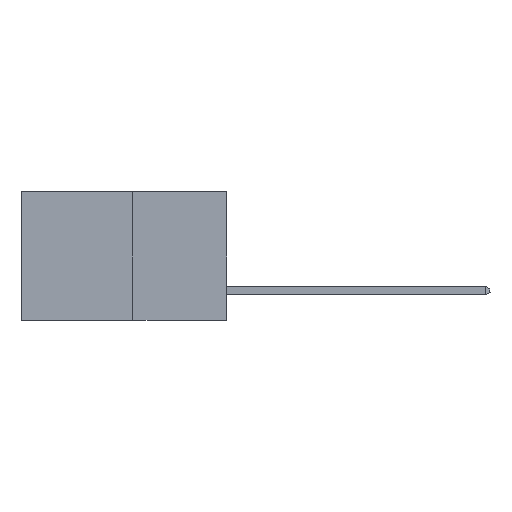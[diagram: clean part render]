
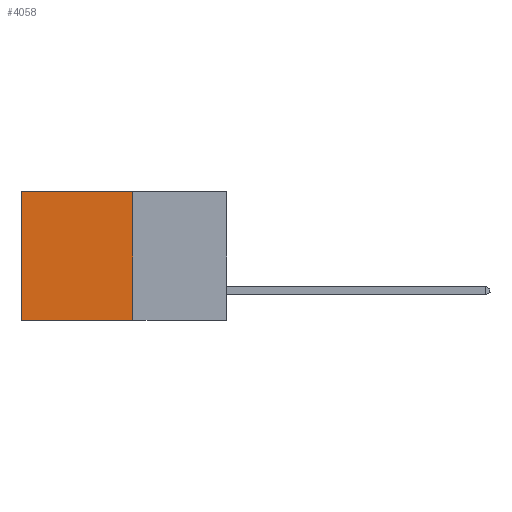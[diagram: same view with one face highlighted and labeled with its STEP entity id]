
A CAD part, left-side view. The second image highlights one B-rep face of the part: STEP entity #4058.
In plain terms, the highlighted planar face has unit normal (-1, 0, 0).
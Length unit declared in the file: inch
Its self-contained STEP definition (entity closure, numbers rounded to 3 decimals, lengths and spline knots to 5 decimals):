
#141 = CARTESIAN_POINT ( 'NONE',  ( 0.277, 0.59, 0. ) ) ;
#2171 = CARTESIAN_POINT ( 'NONE',  ( 0.277, 0.27, 0. ) ) ;
#2784 = VECTOR ( 'NONE', #7173, 39.37008 ) ;
#4058 = ADVANCED_FACE ( 'NONE', ( #8929 ), #28947, .F. ) ;
#4300 = EDGE_CURVE ( 'NONE', #28720, #6236, #8513, .T. ) ;
#4923 = ORIENTED_EDGE ( 'NONE', *, *, #13989, .T. ) ;
#6236 = VERTEX_POINT ( 'NONE', #17850 ) ;
#7173 = DIRECTION ( 'NONE',  ( 0., 1., 0. ) ) ;
#7540 = DIRECTION ( 'NONE',  ( 0., 0., -1. ) ) ;
#7547 = DIRECTION ( 'NONE',  ( 1., 0., 0. ) ) ;
#8355 = VECTOR ( 'NONE', #17525, 39.37008 ) ;
#8513 = LINE ( 'NONE', #13047, #2784 ) ;
#8929 = FACE_OUTER_BOUND ( 'NONE', #14458, .T. ) ;
#8979 = VECTOR ( 'NONE', #29089, 39.37008 ) ;
#9143 = LINE ( 'NONE', #15182, #8355 ) ;
#9300 = ORIENTED_EDGE ( 'NONE', *, *, #25645, .F. ) ;
#11284 = VECTOR ( 'NONE', #19034, 39.37008 ) ;
#11426 = ORIENTED_EDGE ( 'NONE', *, *, #22081, .T. ) ;
#13047 = CARTESIAN_POINT ( 'NONE',  ( 0.277, 0.27, -0.37 ) ) ;
#13196 = VERTEX_POINT ( 'NONE', #141 ) ;
#13989 = EDGE_CURVE ( 'NONE', #19200, #13196, #30146, .T. ) ;
#14458 = EDGE_LOOP ( 'NONE', ( #11426, #21713, #9300, #4923 ) ) ;
#15182 = CARTESIAN_POINT ( 'NONE',  ( 0.277, 0.59, -0.37 ) ) ;
#15570 = CARTESIAN_POINT ( 'NONE',  ( 0.277, 0.27, -0.37 ) ) ;
#17525 = DIRECTION ( 'NONE',  ( 0., 0., -1. ) ) ;
#17850 = CARTESIAN_POINT ( 'NONE',  ( 0.277, 0.59, -0.37 ) ) ;
#19034 = DIRECTION ( 'NONE',  ( 0., 1., 0. ) ) ;
#19200 = VERTEX_POINT ( 'NONE', #23843 ) ;
#21713 = ORIENTED_EDGE ( 'NONE', *, *, #4300, .F. ) ;
#22081 = EDGE_CURVE ( 'NONE', #13196, #6236, #9143, .T. ) ;
#23724 = AXIS2_PLACEMENT_3D ( 'NONE', #15570, #7547, #7540 ) ;
#23843 = CARTESIAN_POINT ( 'NONE',  ( 0.277, 0.27, 0. ) ) ;
#25645 = EDGE_CURVE ( 'NONE', #19200, #28720, #27870, .T. ) ;
#26734 = CARTESIAN_POINT ( 'NONE',  ( 0.277, 0.27, -0.37 ) ) ;
#27870 = LINE ( 'NONE', #26734, #8979 ) ;
#28602 = CARTESIAN_POINT ( 'NONE',  ( 0.277, 0.27, -0.37 ) ) ;
#28720 = VERTEX_POINT ( 'NONE', #28602 ) ;
#28947 = PLANE ( 'NONE',  #23724 ) ;
#29089 = DIRECTION ( 'NONE',  ( 0., 0., -1. ) ) ;
#30146 = LINE ( 'NONE', #2171, #11284 ) ;
